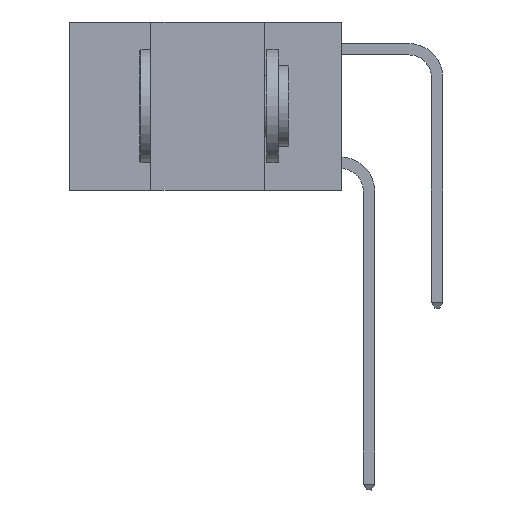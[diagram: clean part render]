
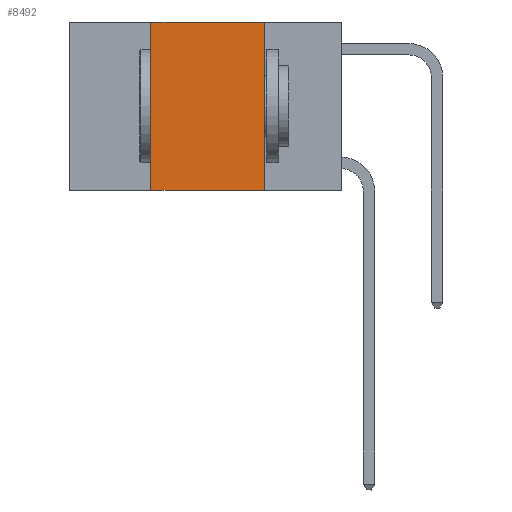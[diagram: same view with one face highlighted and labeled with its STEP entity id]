
A CAD part, left-side view. The second image highlights one B-rep face of the part: STEP entity #8492.
In plain terms, the highlighted planar face has unit normal (-1, 0, 0).
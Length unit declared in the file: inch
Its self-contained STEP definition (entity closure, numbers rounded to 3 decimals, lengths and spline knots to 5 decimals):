
#82 = LINE ( 'NONE', #15255, #17577 ) ;
#353 = EDGE_LOOP ( 'NONE', ( #12416, #11143, #10947, #4232 ) ) ;
#662 = VECTOR ( 'NONE', #8810, 39.37008 ) ;
#1274 = DIRECTION ( 'NONE',  ( 1., 0., 0. ) ) ;
#1393 = CARTESIAN_POINT ( 'NONE',  ( 0., 0.6, 0. ) ) ;
#1780 = VECTOR ( 'NONE', #8507, 39.37008 ) ;
#2093 = VERTEX_POINT ( 'NONE', #13790 ) ;
#2626 = AXIS2_PLACEMENT_3D ( 'NONE', #1393, #1274, #4046 ) ;
#2727 = PLANE ( 'NONE',  #2626 ) ;
#2877 = EDGE_CURVE ( 'NONE', #10613, #16099, #6586, .T. ) ;
#4046 = DIRECTION ( 'NONE',  ( 0., 0., -1. ) ) ;
#4232 = ORIENTED_EDGE ( 'NONE', *, *, #2877, .T. ) ;
#4790 = CARTESIAN_POINT ( 'NONE',  ( 0., 0.6, 0. ) ) ;
#5442 = CARTESIAN_POINT ( 'NONE',  ( 0., 0.42, 0. ) ) ;
#5479 = LINE ( 'NONE', #5442, #1780 ) ;
#6286 = EDGE_CURVE ( 'NONE', #2093, #16099, #82, .T. ) ;
#6586 = LINE ( 'NONE', #7426, #662 ) ;
#7426 = CARTESIAN_POINT ( 'NONE',  ( 0., 0.6, -0.37 ) ) ;
#7514 = DIRECTION ( 'NONE',  ( 0., -1., 0. ) ) ;
#8492 = ADVANCED_FACE ( 'NONE', ( #16335 ), #2727, .F. ) ;
#8507 = DIRECTION ( 'NONE',  ( 0., 0., 1. ) ) ;
#8697 = CARTESIAN_POINT ( 'NONE',  ( 0., 0.42, -0.37 ) ) ;
#8810 = DIRECTION ( 'NONE',  ( 0., -1., 0. ) ) ;
#10005 = EDGE_CURVE ( 'NONE', #10941, #2093, #11889, .T. ) ;
#10613 = VERTEX_POINT ( 'NONE', #8697 ) ;
#10790 = VECTOR ( 'NONE', #7514, 39.37008 ) ;
#10876 = CARTESIAN_POINT ( 'NONE',  ( 0., 0.42, 0. ) ) ;
#10941 = VERTEX_POINT ( 'NONE', #10876 ) ;
#10947 = ORIENTED_EDGE ( 'NONE', *, *, #15883, .F. ) ;
#11143 = ORIENTED_EDGE ( 'NONE', *, *, #10005, .F. ) ;
#11295 = DIRECTION ( 'NONE',  ( 0., 0., -1. ) ) ;
#11434 = CARTESIAN_POINT ( 'NONE',  ( 0., 0.17, -0.37 ) ) ;
#11889 = LINE ( 'NONE', #4790, #10790 ) ;
#12416 = ORIENTED_EDGE ( 'NONE', *, *, #6286, .F. ) ;
#13790 = CARTESIAN_POINT ( 'NONE',  ( 0., 0.17, 0. ) ) ;
#15255 = CARTESIAN_POINT ( 'NONE',  ( 0., 0.17, 0. ) ) ;
#15883 = EDGE_CURVE ( 'NONE', #10613, #10941, #5479, .T. ) ;
#16099 = VERTEX_POINT ( 'NONE', #11434 ) ;
#16335 = FACE_OUTER_BOUND ( 'NONE', #353, .T. ) ;
#17577 = VECTOR ( 'NONE', #11295, 39.37008 ) ;
